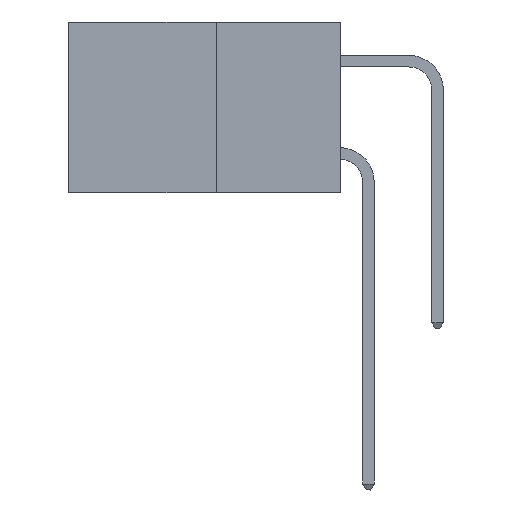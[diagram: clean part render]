
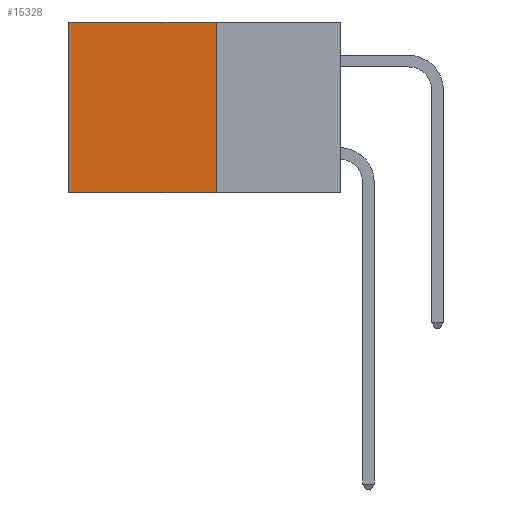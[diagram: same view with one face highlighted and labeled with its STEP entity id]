
A CAD part, left-side view. The second image highlights one B-rep face of the part: STEP entity #15328.
In plain terms, the highlighted planar face has unit normal (-1, 0, 0).
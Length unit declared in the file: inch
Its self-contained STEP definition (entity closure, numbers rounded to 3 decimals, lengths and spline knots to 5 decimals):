
#65 = LINE ( 'NONE', #8157, #2146 ) ;
#294 = CARTESIAN_POINT ( 'NONE',  ( 0.277, 0.27, -0.37 ) ) ;
#654 = ORIENTED_EDGE ( 'NONE', *, *, #8726, .F. ) ;
#898 = ORIENTED_EDGE ( 'NONE', *, *, #16408, .T. ) ;
#1728 = CARTESIAN_POINT ( 'NONE',  ( 0.277, 0.27, -0.37 ) ) ;
#1952 = DIRECTION ( 'NONE',  ( 0., 0., -1. ) ) ;
#2146 = VECTOR ( 'NONE', #9604, 39.37008 ) ;
#2953 = EDGE_CURVE ( 'NONE', #4010, #14495, #13843, .T. ) ;
#3243 = DIRECTION ( 'NONE',  ( 0., 1., 0. ) ) ;
#4010 = VERTEX_POINT ( 'NONE', #14600 ) ;
#4282 = VERTEX_POINT ( 'NONE', #9403 ) ;
#6098 = VECTOR ( 'NONE', #18268, 39.37008 ) ;
#6391 = CARTESIAN_POINT ( 'NONE',  ( 0.277, 0.27, -0.37 ) ) ;
#7732 = CARTESIAN_POINT ( 'NONE',  ( 0.277, 0.59, -0.37 ) ) ;
#7815 = VERTEX_POINT ( 'NONE', #7732 ) ;
#8157 = CARTESIAN_POINT ( 'NONE',  ( 0.277, 0.27, 0. ) ) ;
#8726 = EDGE_CURVE ( 'NONE', #14495, #7815, #15856, .T. ) ;
#8761 = ORIENTED_EDGE ( 'NONE', *, *, #10900, .T. ) ;
#9202 = PLANE ( 'NONE',  #17658 ) ;
#9403 = CARTESIAN_POINT ( 'NONE',  ( 0.277, 0.59, 0. ) ) ;
#9604 = DIRECTION ( 'NONE',  ( 0., 1., 0. ) ) ;
#10542 = VECTOR ( 'NONE', #14494, 39.37008 ) ;
#10634 = DIRECTION ( 'NONE',  ( 1., 0., 0. ) ) ;
#10900 = EDGE_CURVE ( 'NONE', #4010, #4282, #65, .T. ) ;
#13268 = EDGE_LOOP ( 'NONE', ( #898, #654, #16794, #8761 ) ) ;
#13843 = LINE ( 'NONE', #294, #10542 ) ;
#14356 = CARTESIAN_POINT ( 'NONE',  ( 0.277, 0.27, -0.37 ) ) ;
#14494 = DIRECTION ( 'NONE',  ( 0., 0., -1. ) ) ;
#14495 = VERTEX_POINT ( 'NONE', #14356 ) ;
#14600 = CARTESIAN_POINT ( 'NONE',  ( 0.277, 0.27, 0. ) ) ;
#15328 = ADVANCED_FACE ( 'NONE', ( #16666 ), #9202, .F. ) ;
#15420 = VECTOR ( 'NONE', #3243, 39.37008 ) ;
#15497 = CARTESIAN_POINT ( 'NONE',  ( 0.277, 0.59, -0.37 ) ) ;
#15856 = LINE ( 'NONE', #1728, #15420 ) ;
#16408 = EDGE_CURVE ( 'NONE', #4282, #7815, #17278, .T. ) ;
#16666 = FACE_OUTER_BOUND ( 'NONE', #13268, .T. ) ;
#16794 = ORIENTED_EDGE ( 'NONE', *, *, #2953, .F. ) ;
#17278 = LINE ( 'NONE', #15497, #6098 ) ;
#17658 = AXIS2_PLACEMENT_3D ( 'NONE', #6391, #10634, #1952 ) ;
#18268 = DIRECTION ( 'NONE',  ( 0., 0., -1. ) ) ;
